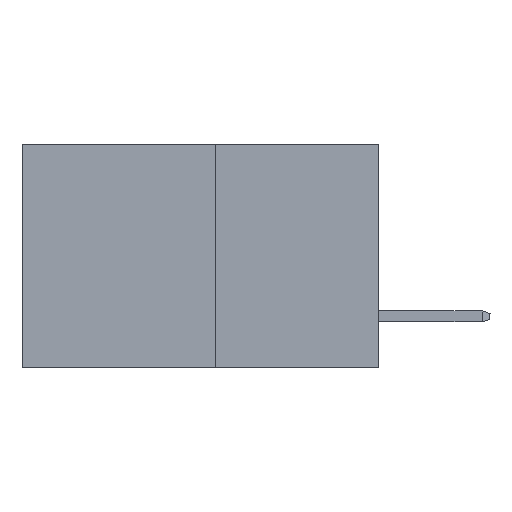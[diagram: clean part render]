
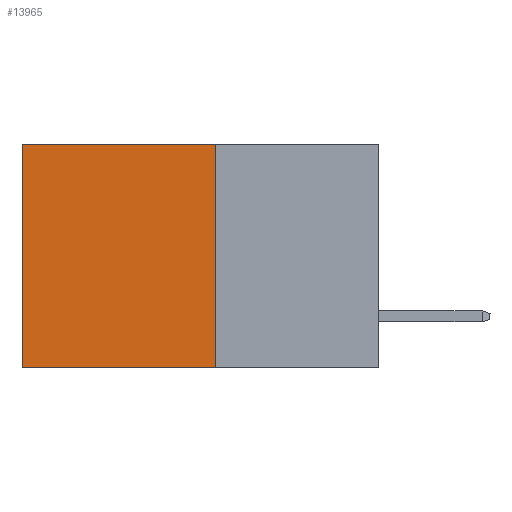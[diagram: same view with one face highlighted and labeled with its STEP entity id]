
A CAD part, left-side view. The second image highlights one B-rep face of the part: STEP entity #13965.
In plain terms, the highlighted planar face has unit normal (-1, 0, 0).
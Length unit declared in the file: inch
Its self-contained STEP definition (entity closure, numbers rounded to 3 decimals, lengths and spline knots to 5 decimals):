
#163 = DIRECTION ( 'NONE',  ( 0., 1., 0. ) ) ;
#198 = EDGE_CURVE ( 'NONE', #9515, #12307, #9493, .T. ) ;
#662 = PLANE ( 'NONE',  #11096 ) ;
#724 = DIRECTION ( 'NONE',  ( 1., 0., 0. ) ) ;
#886 = EDGE_CURVE ( 'NONE', #9247, #13710, #5658, .T. ) ;
#1920 = CARTESIAN_POINT ( 'NONE',  ( 0.277, 0.59, 0. ) ) ;
#1981 = CARTESIAN_POINT ( 'NONE',  ( 0.277, 0.27, -0.37 ) ) ;
#2014 = EDGE_CURVE ( 'NONE', #9515, #9247, #5813, .T. ) ;
#2154 = ORIENTED_EDGE ( 'NONE', *, *, #198, .T. ) ;
#2207 = CARTESIAN_POINT ( 'NONE',  ( 0.277, 0.59, -0.37 ) ) ;
#2361 = VECTOR ( 'NONE', #163, 39.37008 ) ;
#2840 = DIRECTION ( 'NONE',  ( 0., 0., -1. ) ) ;
#2910 = CARTESIAN_POINT ( 'NONE',  ( 0.277, 0.27, -0.37 ) ) ;
#4630 = VECTOR ( 'NONE', #9575, 39.37008 ) ;
#5118 = EDGE_LOOP ( 'NONE', ( #5659, #9245, #10212, #2154 ) ) ;
#5658 = LINE ( 'NONE', #1981, #2361 ) ;
#5659 = ORIENTED_EDGE ( 'NONE', *, *, #5811, .T. ) ;
#5811 = EDGE_CURVE ( 'NONE', #12307, #13710, #10725, .T. ) ;
#5813 = LINE ( 'NONE', #2910, #11831 ) ;
#6154 = DIRECTION ( 'NONE',  ( 0., 1., 0. ) ) ;
#6634 = VECTOR ( 'NONE', #6154, 39.37008 ) ;
#7148 = CARTESIAN_POINT ( 'NONE',  ( 0.277, 0.27, -0.37 ) ) ;
#9245 = ORIENTED_EDGE ( 'NONE', *, *, #886, .F. ) ;
#9247 = VERTEX_POINT ( 'NONE', #7148 ) ;
#9338 = DIRECTION ( 'NONE',  ( 0., 0., -1. ) ) ;
#9493 = LINE ( 'NONE', #10667, #6634 ) ;
#9515 = VERTEX_POINT ( 'NONE', #13494 ) ;
#9575 = DIRECTION ( 'NONE',  ( 0., 0., -1. ) ) ;
#10212 = ORIENTED_EDGE ( 'NONE', *, *, #2014, .F. ) ;
#10483 = FACE_OUTER_BOUND ( 'NONE', #5118, .T. ) ;
#10494 = CARTESIAN_POINT ( 'NONE',  ( 0.277, 0.27, -0.37 ) ) ;
#10667 = CARTESIAN_POINT ( 'NONE',  ( 0.277, 0.27, 0. ) ) ;
#10725 = LINE ( 'NONE', #2207, #4630 ) ;
#11096 = AXIS2_PLACEMENT_3D ( 'NONE', #10494, #724, #9338 ) ;
#11831 = VECTOR ( 'NONE', #2840, 39.37008 ) ;
#12307 = VERTEX_POINT ( 'NONE', #1920 ) ;
#12330 = CARTESIAN_POINT ( 'NONE',  ( 0.277, 0.59, -0.37 ) ) ;
#13494 = CARTESIAN_POINT ( 'NONE',  ( 0.277, 0.27, 0. ) ) ;
#13710 = VERTEX_POINT ( 'NONE', #12330 ) ;
#13965 = ADVANCED_FACE ( 'NONE', ( #10483 ), #662, .F. ) ;
